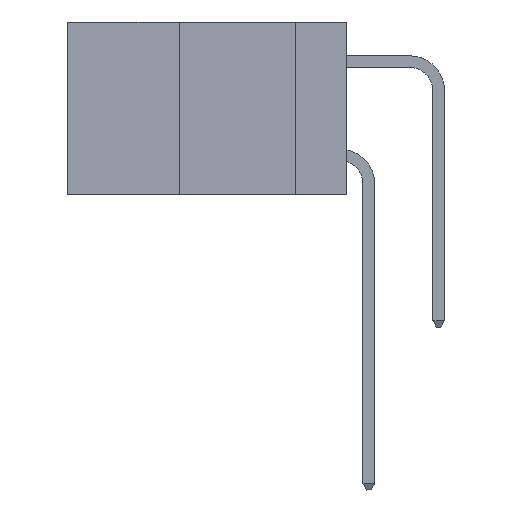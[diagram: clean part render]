
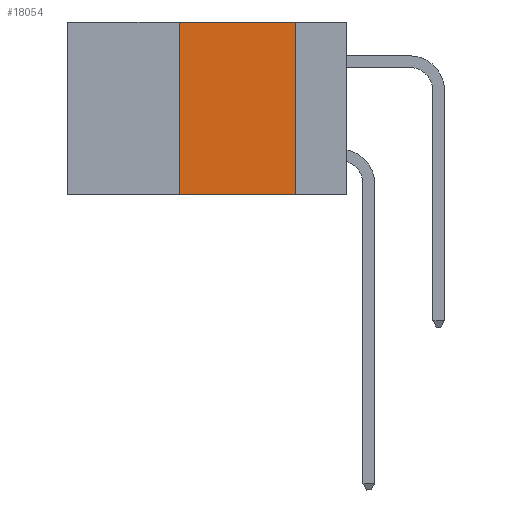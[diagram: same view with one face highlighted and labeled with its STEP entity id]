
A CAD part, left-side view. The second image highlights one B-rep face of the part: STEP entity #18054.
In plain terms, the highlighted planar face has unit normal (-1, 0, 0).
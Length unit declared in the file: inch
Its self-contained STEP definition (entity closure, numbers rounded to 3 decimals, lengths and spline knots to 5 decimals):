
#862 = VECTOR ( 'NONE', #1735, 39.37008 ) ;
#900 = VERTEX_POINT ( 'NONE', #8036 ) ;
#1381 = DIRECTION ( 'NONE',  ( 0., -1., 0. ) ) ;
#1562 = LINE ( 'NONE', #4585, #14350 ) ;
#1735 = DIRECTION ( 'NONE',  ( 0., 0., 1. ) ) ;
#1958 = CARTESIAN_POINT ( 'NONE',  ( 0., 0.36, 0. ) ) ;
#4130 = DIRECTION ( 'NONE',  ( 0., -1., 0. ) ) ;
#4585 = CARTESIAN_POINT ( 'NONE',  ( 0., 0.6, -0.37 ) ) ;
#4614 = VERTEX_POINT ( 'NONE', #21216 ) ;
#5417 = VECTOR ( 'NONE', #17589, 39.37008 ) ;
#6431 = EDGE_CURVE ( 'NONE', #14721, #4614, #14502, .T. ) ;
#7221 = AXIS2_PLACEMENT_3D ( 'NONE', #19306, #11002, #12524 ) ;
#7395 = ORIENTED_EDGE ( 'NONE', *, *, #20003, .F. ) ;
#8036 = CARTESIAN_POINT ( 'NONE',  ( 0., 0.11, -0.37 ) ) ;
#8965 = EDGE_CURVE ( 'NONE', #17288, #14721, #20995, .T. ) ;
#9225 = PLANE ( 'NONE',  #7221 ) ;
#9326 = LINE ( 'NONE', #10891, #5417 ) ;
#9848 = CARTESIAN_POINT ( 'NONE',  ( 0., 0.36, -0.37 ) ) ;
#10085 = VECTOR ( 'NONE', #4130, 39.37008 ) ;
#10891 = CARTESIAN_POINT ( 'NONE',  ( 0., 0.11, 0. ) ) ;
#11002 = DIRECTION ( 'NONE',  ( 1., 0., 0. ) ) ;
#11053 = CARTESIAN_POINT ( 'NONE',  ( 0., 0.36, 0. ) ) ;
#12524 = DIRECTION ( 'NONE',  ( 0., 0., -1. ) ) ;
#14350 = VECTOR ( 'NONE', #1381, 39.37008 ) ;
#14502 = LINE ( 'NONE', #15747, #10085 ) ;
#14721 = VERTEX_POINT ( 'NONE', #11053 ) ;
#15747 = CARTESIAN_POINT ( 'NONE',  ( 0., 0.6, 0. ) ) ;
#17288 = VERTEX_POINT ( 'NONE', #9848 ) ;
#17589 = DIRECTION ( 'NONE',  ( 0., 0., -1. ) ) ;
#17647 = EDGE_CURVE ( 'NONE', #17288, #900, #1562, .T. ) ;
#18054 = ADVANCED_FACE ( 'NONE', ( #20623 ), #9225, .F. ) ;
#18091 = EDGE_LOOP ( 'NONE', ( #7395, #20129, #20399, #18716 ) ) ;
#18716 = ORIENTED_EDGE ( 'NONE', *, *, #17647, .T. ) ;
#19306 = CARTESIAN_POINT ( 'NONE',  ( 0., 0.6, 0. ) ) ;
#20003 = EDGE_CURVE ( 'NONE', #4614, #900, #9326, .T. ) ;
#20129 = ORIENTED_EDGE ( 'NONE', *, *, #6431, .F. ) ;
#20399 = ORIENTED_EDGE ( 'NONE', *, *, #8965, .F. ) ;
#20623 = FACE_OUTER_BOUND ( 'NONE', #18091, .T. ) ;
#20995 = LINE ( 'NONE', #1958, #862 ) ;
#21216 = CARTESIAN_POINT ( 'NONE',  ( 0., 0.11, 0. ) ) ;
